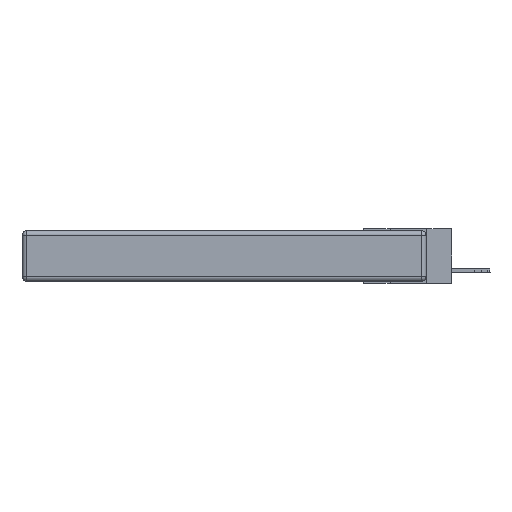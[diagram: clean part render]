
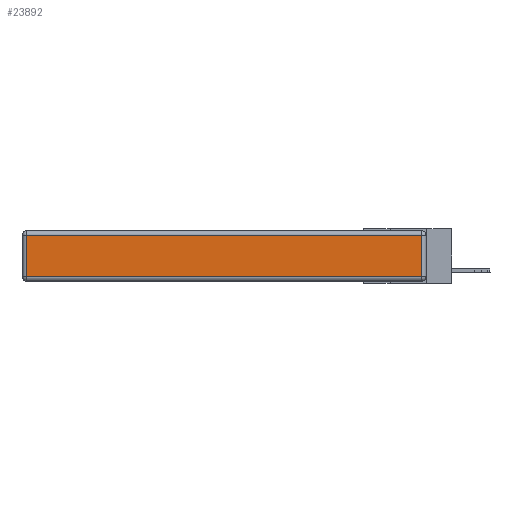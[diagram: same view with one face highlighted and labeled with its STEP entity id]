
A CAD part, left-side view. The second image highlights one B-rep face of the part: STEP entity #23892.
In plain terms, the highlighted planar face has unit normal (-1, 0, 0).
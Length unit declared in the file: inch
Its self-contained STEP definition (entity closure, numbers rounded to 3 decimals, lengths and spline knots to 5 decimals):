
#137 = CARTESIAN_POINT ( 'NONE',  ( 0., 0., -0.313 ) ) ;
#151 = EDGE_CURVE ( 'NONE', #5365, #6358, #2779, .T. ) ;
#172 = CARTESIAN_POINT ( 'NONE',  ( 0., 0.03, -0.343 ) ) ;
#621 = DIRECTION ( 'NONE',  ( 0., 0., 1. ) ) ;
#650 = DIRECTION ( 'NONE',  ( 0., 1., 0. ) ) ;
#1935 = VERTEX_POINT ( 'NONE', #10999 ) ;
#1986 = CARTESIAN_POINT ( 'NONE',  ( 0., 0.03, -0.03 ) ) ;
#2206 = CARTESIAN_POINT ( 'NONE',  ( 0., 2.72, -0.03 ) ) ;
#2451 = DIRECTION ( 'NONE',  ( 0., -1., 0. ) ) ;
#2482 = VECTOR ( 'NONE', #650, 39.37008 ) ;
#2744 = EDGE_CURVE ( 'NONE', #1935, #21714, #4356, .T. ) ;
#2779 = LINE ( 'NONE', #8490, #2482 ) ;
#4356 = LINE ( 'NONE', #137, #16369 ) ;
#5123 = FACE_OUTER_BOUND ( 'NONE', #13370, .T. ) ;
#5365 = VERTEX_POINT ( 'NONE', #1986 ) ;
#5373 = VECTOR ( 'NONE', #11723, 39.37008 ) ;
#6358 = VERTEX_POINT ( 'NONE', #2206 ) ;
#6529 = PLANE ( 'NONE',  #11735 ) ;
#6832 = VECTOR ( 'NONE', #23757, 39.37008 ) ;
#7901 = ORIENTED_EDGE ( 'NONE', *, *, #2744, .T. ) ;
#8387 = CARTESIAN_POINT ( 'NONE',  ( 0., 2.72, -0.343 ) ) ;
#8490 = CARTESIAN_POINT ( 'NONE',  ( 0., 2.75, -0.03 ) ) ;
#9676 = EDGE_CURVE ( 'NONE', #21714, #5365, #14100, .T. ) ;
#10147 = DIRECTION ( 'NONE',  ( -1., 0., 0. ) ) ;
#10784 = EDGE_CURVE ( 'NONE', #6358, #1935, #20966, .T. ) ;
#10999 = CARTESIAN_POINT ( 'NONE',  ( 0., 2.72, -0.313 ) ) ;
#11723 = DIRECTION ( 'NONE',  ( 0., 0., 1. ) ) ;
#11735 = AXIS2_PLACEMENT_3D ( 'NONE', #21645, #10147, #621 ) ;
#13370 = EDGE_LOOP ( 'NONE', ( #7901, #17034, #24525, #17362 ) ) ;
#14100 = LINE ( 'NONE', #172, #5373 ) ;
#16369 = VECTOR ( 'NONE', #2451, 39.37008 ) ;
#17034 = ORIENTED_EDGE ( 'NONE', *, *, #9676, .T. ) ;
#17362 = ORIENTED_EDGE ( 'NONE', *, *, #10784, .T. ) ;
#20966 = LINE ( 'NONE', #8387, #6832 ) ;
#21362 = CARTESIAN_POINT ( 'NONE',  ( 0., 0.03, -0.313 ) ) ;
#21645 = CARTESIAN_POINT ( 'NONE',  ( 0., 0., -0.343 ) ) ;
#21714 = VERTEX_POINT ( 'NONE', #21362 ) ;
#23757 = DIRECTION ( 'NONE',  ( 0., 0., -1. ) ) ;
#23892 = ADVANCED_FACE ( 'NONE', ( #5123 ), #6529, .T. ) ;
#24525 = ORIENTED_EDGE ( 'NONE', *, *, #151, .T. ) ;
